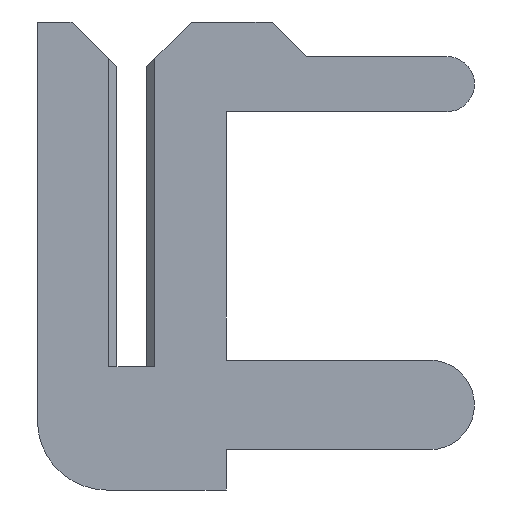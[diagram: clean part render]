
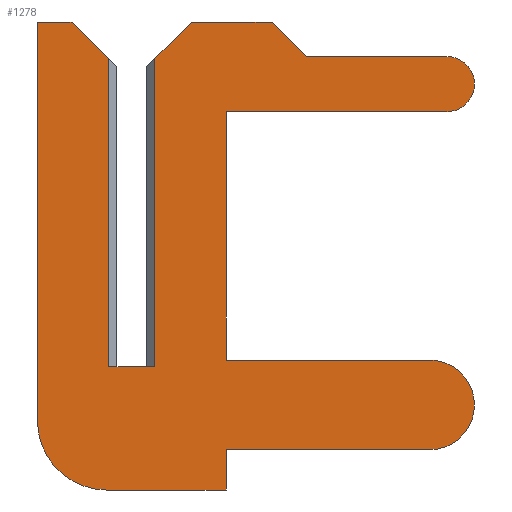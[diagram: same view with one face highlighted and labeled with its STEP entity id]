
A CAD part, left-side view. The second image highlights one B-rep face of the part: STEP entity #1278.
In plain terms, the highlighted planar face has unit normal (-1, 0, 0).
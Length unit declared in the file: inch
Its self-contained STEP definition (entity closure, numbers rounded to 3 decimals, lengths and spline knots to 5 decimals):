
#1 = VERTEX_POINT ( 'NONE', #1044 ) ;
#10 = VECTOR ( 'NONE', #616, 39.37008 ) ;
#24 = ORIENTED_EDGE ( 'NONE', *, *, #653, .F. ) ;
#25 = DIRECTION ( 'NONE',  ( 0., 0., 1. ) ) ;
#30 = VECTOR ( 'NONE', #401, 39.37008 ) ;
#36 = ORIENTED_EDGE ( 'NONE', *, *, #1755, .F. ) ;
#48 = DIRECTION ( 'NONE',  ( 0., -0.707, -0.707 ) ) ;
#78 = ORIENTED_EDGE ( 'NONE', *, *, #390, .F. ) ;
#87 = VERTEX_POINT ( 'NONE', #480 ) ;
#89 = VECTOR ( 'NONE', #48, 39.37008 ) ;
#106 = EDGE_CURVE ( 'NONE', #130, #1403, #806, .T. ) ;
#109 = DIRECTION ( 'NONE',  ( 1., 0., 0. ) ) ;
#115 = CIRCLE ( 'NONE', #1120, 0.012 ) ;
#117 = ORIENTED_EDGE ( 'NONE', *, *, #359, .F. ) ;
#130 = VERTEX_POINT ( 'NONE', #320 ) ;
#132 = CIRCLE ( 'NONE', #744, 0.0195 ) ;
#142 = VERTEX_POINT ( 'NONE', #603 ) ;
#152 = ORIENTED_EDGE ( 'NONE', *, *, #990, .F. ) ;
#154 = ORIENTED_EDGE ( 'NONE', *, *, #106, .F. ) ;
#180 = DIRECTION ( 'NONE',  ( 0., 1., 0. ) ) ;
#183 = ORIENTED_EDGE ( 'NONE', *, *, #893, .F. ) ;
#186 = CARTESIAN_POINT ( 'NONE',  ( -0.01, 0.041, 0.15 ) ) ;
#194 = CARTESIAN_POINT ( 'NONE',  ( -0.01, -0.1295, 0.003 ) ) ;
#201 = EDGE_CURVE ( 'NONE', #828, #422, #961, .T. ) ;
#211 = EDGE_CURVE ( 'NONE', #1500, #942, #1081, .T. ) ;
#236 = VERTEX_POINT ( 'NONE', #774 ) ;
#247 = ORIENTED_EDGE ( 'NONE', *, *, #1390, .T. ) ;
#263 = EDGE_CURVE ( 'NONE', #965, #1500, #1766, .T. ) ;
#266 = DIRECTION ( 'NONE',  ( 0., -1., 0. ) ) ;
#289 = EDGE_CURVE ( 'NONE', #486, #377, #1359, .T. ) ;
#309 = CARTESIAN_POINT ( 'NONE',  ( -0.01, -0.041, 0.003 ) ) ;
#318 = DIRECTION ( 'NONE',  ( 0., -1., 0. ) ) ;
#320 = CARTESIAN_POINT ( 'NONE',  ( -0.01, -0.137, 0.111 ) ) ;
#329 = VECTOR ( 'NONE', #741, 39.37008 ) ;
#343 = CARTESIAN_POINT ( 'NONE',  ( -0.01, 0.01, 0.134 ) ) ;
#359 = EDGE_CURVE ( 'NONE', #1, #1512, #622, .T. ) ;
#377 = VERTEX_POINT ( 'NONE', #1665 ) ;
#390 = EDGE_CURVE ( 'NONE', #1380, #1, #1329, .T. ) ;
#391 = CARTESIAN_POINT ( 'NONE',  ( -0.01, 0.011, -0.0235 ) ) ;
#393 = ORIENTED_EDGE ( 'NONE', *, *, #416, .F. ) ;
#395 = VECTOR ( 'NONE', #180, 39.37008 ) ;
#401 = DIRECTION ( 'NONE',  ( 0., -1., 0. ) ) ;
#405 = AXIS2_PLACEMENT_3D ( 'NONE', #391, #109, #580 ) ;
#409 = VECTOR ( 'NONE', #318, 39.37008 ) ;
#416 = EDGE_CURVE ( 'NONE', #422, #965, #1649, .T. ) ;
#422 = VERTEX_POINT ( 'NONE', #572 ) ;
#436 = LINE ( 'NONE', #1140, #409 ) ;
#439 = DIRECTION ( 'NONE',  ( 0., 0., -1. ) ) ;
#465 = DIRECTION ( 'NONE',  ( 0., -1., 0. ) ) ;
#475 = CARTESIAN_POINT ( 'NONE',  ( -0.01, -0.137, 0.123 ) ) ;
#478 = VECTOR ( 'NONE', #1268, 39.37008 ) ;
#480 = CARTESIAN_POINT ( 'NONE',  ( -0.01, 0.026, 0.15 ) ) ;
#485 = VERTEX_POINT ( 'NONE', #716 ) ;
#486 = VERTEX_POINT ( 'NONE', #1676 ) ;
#541 = LINE ( 'NONE', #1559, #89 ) ;
#572 = CARTESIAN_POINT ( 'NONE',  ( -0.01, -0.026, 0.15 ) ) ;
#580 = DIRECTION ( 'NONE',  ( 0., 0., 1. ) ) ;
#588 = DIRECTION ( 'NONE',  ( -1., 0., 0. ) ) ;
#595 = VECTOR ( 'NONE', #266, 39.37008 ) ;
#596 = VECTOR ( 'NONE', #1203, 39.37008 ) ;
#603 = CARTESIAN_POINT ( 'NONE',  ( -0.01, 0.01, 0. ) ) ;
#612 = CARTESIAN_POINT ( 'NONE',  ( -0.01, -0.041, -0.036 ) ) ;
#616 = DIRECTION ( 'NONE',  ( 0., 1., 0. ) ) ;
#619 = AXIS2_PLACEMENT_3D ( 'NONE', #733, #588, #1436 ) ;
#622 = LINE ( 'NONE', #671, #825 ) ;
#642 = EDGE_CURVE ( 'NONE', #142, #1187, #1696, .T. ) ;
#651 = ORIENTED_EDGE ( 'NONE', *, *, #1535, .F. ) ;
#653 = EDGE_CURVE ( 'NONE', #1010, #816, #132, .T. ) ;
#671 = CARTESIAN_POINT ( 'NONE',  ( -0.01, 0.041, 0.15 ) ) ;
#672 = ORIENTED_EDGE ( 'NONE', *, *, #1569, .F. ) ;
#700 = LINE ( 'NONE', #1007, #1055 ) ;
#704 = VECTOR ( 'NONE', #1606, 39.37008 ) ;
#716 = CARTESIAN_POINT ( 'NONE',  ( -0.01, -0.041, 0.003 ) ) ;
#725 = LINE ( 'NONE', #891, #1701 ) ;
#726 = CARTESIAN_POINT ( 'NONE',  ( -0.01, 0.011, -0.0535 ) ) ;
#733 = CARTESIAN_POINT ( 'NONE',  ( -0.01, 0.011, -0.0235 ) ) ;
#737 = CARTESIAN_POINT ( 'NONE',  ( -0.01, -0.01, 0.134 ) ) ;
#741 = DIRECTION ( 'NONE',  ( 0., 0., -1. ) ) ;
#744 = AXIS2_PLACEMENT_3D ( 'NONE', #1540, #846, #25 ) ;
#755 = DIRECTION ( 'NONE',  ( 1., 0., 0. ) ) ;
#769 = ORIENTED_EDGE ( 'NONE', *, *, #642, .T. ) ;
#774 = CARTESIAN_POINT ( 'NONE',  ( -0.01, -0.01, 0. ) ) ;
#780 = DIRECTION ( 'NONE',  ( 0., -0.707, -0.707 ) ) ;
#806 = LINE ( 'NONE', #890, #395 ) ;
#816 = VERTEX_POINT ( 'NONE', #1440 ) ;
#825 = VECTOR ( 'NONE', #1636, 39.37008 ) ;
#828 = VERTEX_POINT ( 'NONE', #737 ) ;
#846 = DIRECTION ( 'NONE',  ( 1., 0., 0. ) ) ;
#854 = PLANE ( 'NONE',  #619 ) ;
#881 = CARTESIAN_POINT ( 'NONE',  ( -0.01, 0.011, -0.0535 ) ) ;
#890 = CARTESIAN_POINT ( 'NONE',  ( -0.01, -0.041, 0.111 ) ) ;
#891 = CARTESIAN_POINT ( 'NONE',  ( -0.01, 0.0065, 0. ) ) ;
#893 = EDGE_CURVE ( 'NONE', #87, #1187, #541, .T. ) ;
#931 = ORIENTED_EDGE ( 'NONE', *, *, #211, .F. ) ;
#941 = EDGE_CURVE ( 'NONE', #1512, #87, #436, .T. ) ;
#942 = VERTEX_POINT ( 'NONE', #1553 ) ;
#950 = ORIENTED_EDGE ( 'NONE', *, *, #1662, .F. ) ;
#961 = LINE ( 'NONE', #1198, #596 ) ;
#965 = VERTEX_POINT ( 'NONE', #1300 ) ;
#987 = VECTOR ( 'NONE', #1332, 39.37008 ) ;
#990 = EDGE_CURVE ( 'NONE', #1403, #485, #1542, .T. ) ;
#1007 = CARTESIAN_POINT ( 'NONE',  ( -0.01, -0.01, 0.15 ) ) ;
#1009 = VECTOR ( 'NONE', #1182, 39.37008 ) ;
#1010 = VERTEX_POINT ( 'NONE', #194 ) ;
#1044 = CARTESIAN_POINT ( 'NONE',  ( -0.01, 0.041, -0.0235 ) ) ;
#1055 = VECTOR ( 'NONE', #439, 39.37008 ) ;
#1066 = CARTESIAN_POINT ( 'NONE',  ( -0.01, -0.041, -0.0535 ) ) ;
#1077 = LINE ( 'NONE', #881, #1009 ) ;
#1081 = LINE ( 'NONE', #1474, #704 ) ;
#1117 = LINE ( 'NONE', #1260, #595 ) ;
#1120 = AXIS2_PLACEMENT_3D ( 'NONE', #475, #755, #1319 ) ;
#1140 = CARTESIAN_POINT ( 'NONE',  ( -0.01, 0.026, 0.15 ) ) ;
#1144 = ORIENTED_EDGE ( 'NONE', *, *, #941, .F. ) ;
#1161 = CARTESIAN_POINT ( 'NONE',  ( -0.01, -0.026, 0.15 ) ) ;
#1182 = DIRECTION ( 'NONE',  ( 0., 1., 0. ) ) ;
#1187 = VERTEX_POINT ( 'NONE', #343 ) ;
#1197 = CARTESIAN_POINT ( 'NONE',  ( -0.01, -0.076, 0.135 ) ) ;
#1198 = CARTESIAN_POINT ( 'NONE',  ( -0.01, -0.0065, 0.1305 ) ) ;
#1203 = DIRECTION ( 'NONE',  ( 0., -0.707, 0.707 ) ) ;
#1218 = ORIENTED_EDGE ( 'NONE', *, *, #1599, .F. ) ;
#1249 = CARTESIAN_POINT ( 'NONE',  ( -0.01, 0.01, -0.0235 ) ) ;
#1260 = CARTESIAN_POINT ( 'NONE',  ( -0.01, -0.1295, 0.003 ) ) ;
#1268 = DIRECTION ( 'NONE',  ( 0., 0., 1. ) ) ;
#1278 = ADVANCED_FACE ( 'NONE', ( #1401 ), #854, .T. ) ;
#1289 = CARTESIAN_POINT ( 'NONE',  ( -0.01, -0.041, 0.111 ) ) ;
#1300 = CARTESIAN_POINT ( 'NONE',  ( -0.01, -0.061, 0.15 ) ) ;
#1319 = DIRECTION ( 'NONE',  ( 0., 0., 1. ) ) ;
#1329 = CIRCLE ( 'NONE', #405, 0.03 ) ;
#1332 = DIRECTION ( 'NONE',  ( 0., 0., -1. ) ) ;
#1359 = LINE ( 'NONE', #1066, #987 ) ;
#1380 = VERTEX_POINT ( 'NONE', #726 ) ;
#1390 = EDGE_CURVE ( 'NONE', #828, #236, #700, .T. ) ;
#1401 = FACE_OUTER_BOUND ( 'NONE', #1475, .T. ) ;
#1403 = VERTEX_POINT ( 'NONE', #1289 ) ;
#1404 = VECTOR ( 'NONE', #780, 39.37008 ) ;
#1406 = ORIENTED_EDGE ( 'NONE', *, *, #289, .F. ) ;
#1436 = DIRECTION ( 'NONE',  ( 0., 0., 1. ) ) ;
#1440 = CARTESIAN_POINT ( 'NONE',  ( -0.01, -0.1295, -0.036 ) ) ;
#1474 = CARTESIAN_POINT ( 'NONE',  ( -0.01, -0.137, 0.135 ) ) ;
#1475 = EDGE_LOOP ( 'NONE', ( #1657, #247, #950, #769, #183, #1144, #117, #78, #1218, #1406, #672, #24, #36, #152, #154, #651, #931, #1644, #393 ) ) ;
#1500 = VERTEX_POINT ( 'NONE', #1561 ) ;
#1512 = VERTEX_POINT ( 'NONE', #186 ) ;
#1535 = EDGE_CURVE ( 'NONE', #942, #130, #115, .T. ) ;
#1540 = CARTESIAN_POINT ( 'NONE',  ( -0.01, -0.1295, -0.0165 ) ) ;
#1542 = LINE ( 'NONE', #309, #329 ) ;
#1553 = CARTESIAN_POINT ( 'NONE',  ( -0.01, -0.137, 0.135 ) ) ;
#1559 = CARTESIAN_POINT ( 'NONE',  ( -0.01, 0.0065, 0.1305 ) ) ;
#1561 = CARTESIAN_POINT ( 'NONE',  ( -0.01, -0.076, 0.135 ) ) ;
#1569 = EDGE_CURVE ( 'NONE', #816, #486, #1570, .T. ) ;
#1570 = LINE ( 'NONE', #612, #10 ) ;
#1599 = EDGE_CURVE ( 'NONE', #377, #1380, #1077, .T. ) ;
#1606 = DIRECTION ( 'NONE',  ( 0., -1., 0. ) ) ;
#1636 = DIRECTION ( 'NONE',  ( 0., 0., 1. ) ) ;
#1644 = ORIENTED_EDGE ( 'NONE', *, *, #263, .F. ) ;
#1649 = LINE ( 'NONE', #1161, #30 ) ;
#1657 = ORIENTED_EDGE ( 'NONE', *, *, #201, .F. ) ;
#1662 = EDGE_CURVE ( 'NONE', #142, #236, #725, .T. ) ;
#1665 = CARTESIAN_POINT ( 'NONE',  ( -0.01, -0.041, -0.0535 ) ) ;
#1676 = CARTESIAN_POINT ( 'NONE',  ( -0.01, -0.041, -0.036 ) ) ;
#1696 = LINE ( 'NONE', #1249, #478 ) ;
#1701 = VECTOR ( 'NONE', #465, 39.37008 ) ;
#1755 = EDGE_CURVE ( 'NONE', #485, #1010, #1117, .T. ) ;
#1766 = LINE ( 'NONE', #1197, #1404 ) ;
